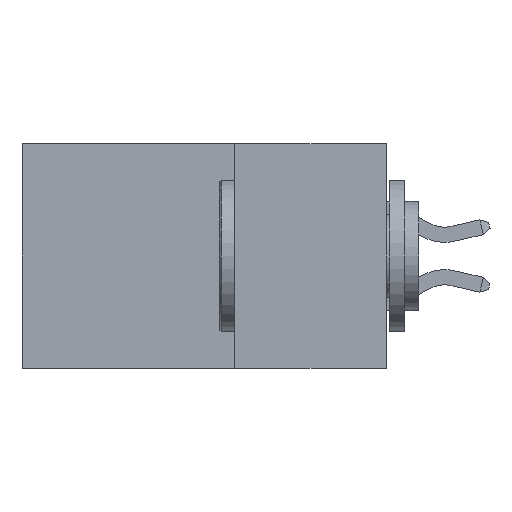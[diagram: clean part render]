
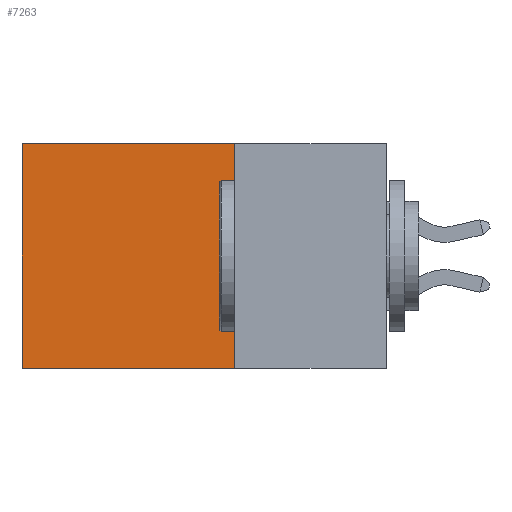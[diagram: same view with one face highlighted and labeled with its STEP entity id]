
A CAD part, left-side view. The second image highlights one B-rep face of the part: STEP entity #7263.
In plain terms, the highlighted planar face has unit normal (-1, 0, 0).
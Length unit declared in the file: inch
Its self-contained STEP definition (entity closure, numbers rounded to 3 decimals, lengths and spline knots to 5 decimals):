
#307 = CARTESIAN_POINT ( 'NONE',  ( 0.298, 0.25, 0. ) ) ;
#2355 = DIRECTION ( 'NONE',  ( 1., 0., 0. ) ) ;
#2365 = PLANE ( 'NONE',  #19147 ) ;
#2661 = CARTESIAN_POINT ( 'NONE',  ( 0.298, 0.6, 0. ) ) ;
#3024 = VECTOR ( 'NONE', #11901, 39.37008 ) ;
#3885 = CARTESIAN_POINT ( 'NONE',  ( 0.298, 0.25, -0.37 ) ) ;
#4986 = ORIENTED_EDGE ( 'NONE', *, *, #14093, .F. ) ;
#6966 = CARTESIAN_POINT ( 'NONE',  ( 0.298, 0.25, 0. ) ) ;
#7263 = ADVANCED_FACE ( 'NONE', ( #24330 ), #2365, .F. ) ;
#7797 = CARTESIAN_POINT ( 'NONE',  ( 0.298, 0.25, -0.37 ) ) ;
#9429 = LINE ( 'NONE', #2661, #26423 ) ;
#10502 = LINE ( 'NONE', #22934, #3024 ) ;
#11426 = DIRECTION ( 'NONE',  ( 0., 0., -1. ) ) ;
#11901 = DIRECTION ( 'NONE',  ( 0., 1., 0. ) ) ;
#11946 = CARTESIAN_POINT ( 'NONE',  ( 0.298, 0.6, 0. ) ) ;
#12358 = EDGE_CURVE ( 'NONE', #19578, #24651, #19878, .T. ) ;
#12520 = EDGE_CURVE ( 'NONE', #19578, #15625, #10502, .T. ) ;
#12790 = VERTEX_POINT ( 'NONE', #19736 ) ;
#13614 = ORIENTED_EDGE ( 'NONE', *, *, #20837, .T. ) ;
#14007 = VECTOR ( 'NONE', #11426, 39.37008 ) ;
#14093 = EDGE_CURVE ( 'NONE', #24651, #12790, #25361, .T. ) ;
#14859 = EDGE_LOOP ( 'NONE', ( #13614, #4986, #25360, #23799 ) ) ;
#15625 = VERTEX_POINT ( 'NONE', #11946 ) ;
#15855 = DIRECTION ( 'NONE',  ( 0., 0., -1. ) ) ;
#16152 = DIRECTION ( 'NONE',  ( 0., 0., -1. ) ) ;
#18024 = CARTESIAN_POINT ( 'NONE',  ( 0.298, 0.25, 0. ) ) ;
#19147 = AXIS2_PLACEMENT_3D ( 'NONE', #307, #2355, #15855 ) ;
#19467 = VECTOR ( 'NONE', #21791, 39.37008 ) ;
#19578 = VERTEX_POINT ( 'NONE', #6966 ) ;
#19736 = CARTESIAN_POINT ( 'NONE',  ( 0.298, 0.6, -0.37 ) ) ;
#19878 = LINE ( 'NONE', #18024, #14007 ) ;
#20837 = EDGE_CURVE ( 'NONE', #15625, #12790, #9429, .T. ) ;
#21791 = DIRECTION ( 'NONE',  ( 0., 1., 0. ) ) ;
#22934 = CARTESIAN_POINT ( 'NONE',  ( 0.298, 0.25, 0. ) ) ;
#23799 = ORIENTED_EDGE ( 'NONE', *, *, #12520, .T. ) ;
#24330 = FACE_OUTER_BOUND ( 'NONE', #14859, .T. ) ;
#24651 = VERTEX_POINT ( 'NONE', #7797 ) ;
#25360 = ORIENTED_EDGE ( 'NONE', *, *, #12358, .F. ) ;
#25361 = LINE ( 'NONE', #3885, #19467 ) ;
#26423 = VECTOR ( 'NONE', #16152, 39.37008 ) ;
